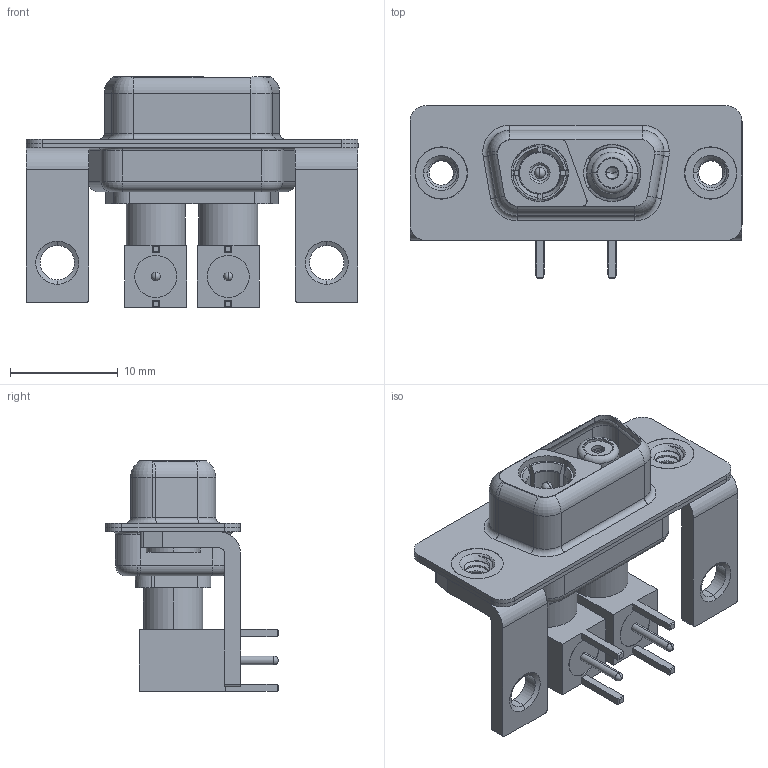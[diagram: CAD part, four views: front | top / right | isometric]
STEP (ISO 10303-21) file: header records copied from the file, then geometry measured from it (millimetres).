
FILE_DESCRIPTION (( 'STEP AP203' ), '1' );
FILE_NAME ('630-2WK2640-7N4.STEP', '2022-05-27T03:34:58', ( '' ), ( '' ), 'SwSTEP 2.0', 'SolidWorks 2020', '' );
FILE_SCHEMA (( 'CONFIG_CONTROL_DESIGN' ));
Length unit declared in the file: millimetre
Products named in the file (18): Co-Ax Plug_RA PC Tail; Co-Ax Jack Assy_RA; 630Combo Threaded Rivet_3; Socket_RA; 630Combo Stabilizer Bracket; Insulator Socket 2; Pin_RA; Co-Ax Jack_RA PC Tail; 630Combo Shell Front_09 Contacts; 630Combo Shell Rear_09 Contacts; 630-2WK2640-7N4; Co-Ax Plug Assy_RA; Insulator Socket; 630Combo Housing_2WK2; Locking Collar; RA Back Shell; Insulator Pin_Straight PC Tail; Insulator RA Pin
Assembly tree (22 placements, depth 3):
  630-2WK2640-7N4
    630Combo Housing_2WK2
    630Combo Shell Front_09 Contacts
    630Combo Shell Rear_09 Contacts
    630Combo Threaded Rivet_3  x2
    630Combo Stabilizer Bracket  x2
    Co-Ax Plug Assy_RA
      Co-Ax Plug_RA PC Tail
      Insulator Pin_Straight PC Tail
      Pin_RA
      Locking Collar
      RA Back Shell
      Insulator RA Pin
    Co-Ax Jack Assy_RA
      Co-Ax Jack_RA PC Tail
      Insulator Socket
      Insulator Socket 2
      Locking Collar
      Socket_RA
      RA Back Shell
      Insulator RA Pin
Bounding box: 30.8 x 16 x 21.41 mm (x, y, z)
Volume: 2278.9 mm3; surface area: 6154.4 mm2
Topology: 20 solids, 20 shells, 640 faces, 1540 edges, 963 vertices
Faces by surface type: cylinder 288, plane 211, torus 69, cone 58, bspline 8, sphere 6
Entity records: 19148 total; most frequent: CARTESIAN_POINT 4470, DIRECTION 2861, ORIENTED_EDGE 2506, EDGE_CURVE 1253, AXIS2_PLACEMENT_3D 1160, VERTEX_POINT 791, CIRCLE 607, EDGE_LOOP 604
